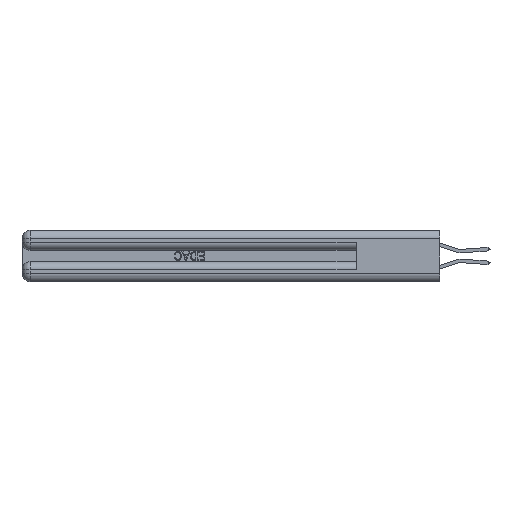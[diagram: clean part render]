
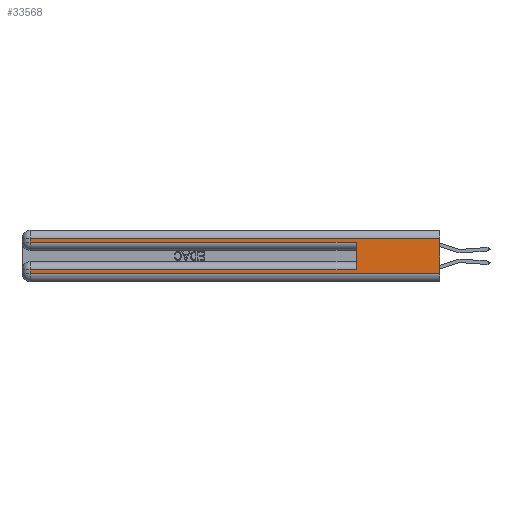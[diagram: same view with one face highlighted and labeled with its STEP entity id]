
A CAD part, left-side view. The second image highlights one B-rep face of the part: STEP entity #33568.
In plain terms, the highlighted planar face has unit normal (-1, 0, 0).
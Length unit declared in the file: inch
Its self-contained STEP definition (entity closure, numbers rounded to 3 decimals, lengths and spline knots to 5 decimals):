
#102 = CARTESIAN_POINT ( 'NONE',  ( 0., 0., 0.37 ) ) ;
#233 = EDGE_CURVE ( 'NONE', #40663, #16151, #23575, .T. ) ;
#331 = EDGE_LOOP ( 'NONE', ( #36158, #1715, #20571, #21414, #36851, #10045, #33916, #22500 ) ) ;
#1715 = ORIENTED_EDGE ( 'NONE', *, *, #34151, .T. ) ;
#2573 = PLANE ( 'NONE',  #15034 ) ;
#2609 = CARTESIAN_POINT ( 'NONE',  ( 0., 0.6, 0.285 ) ) ;
#2810 = VECTOR ( 'NONE', #10468, 39.37008 ) ;
#4701 = VERTEX_POINT ( 'NONE', #22390 ) ;
#4726 = CARTESIAN_POINT ( 'NONE',  ( 0., 0., 0.31 ) ) ;
#4946 = VECTOR ( 'NONE', #12171, 39.37008 ) ;
#5320 = LINE ( 'NONE', #102, #11819 ) ;
#5517 = FACE_OUTER_BOUND ( 'NONE', #331, .T. ) ;
#5545 = VECTOR ( 'NONE', #16810, 39.37008 ) ;
#6520 = CARTESIAN_POINT ( 'NONE',  ( 0., 2.94, 0.085 ) ) ;
#7369 = VERTEX_POINT ( 'NONE', #13444 ) ;
#7971 = VECTOR ( 'NONE', #37276, 39.37008 ) ;
#9285 = CARTESIAN_POINT ( 'NONE',  ( 0., 2.94, 0.31 ) ) ;
#9429 = CARTESIAN_POINT ( 'NONE',  ( 0., 2.94, 0.37 ) ) ;
#10045 = ORIENTED_EDGE ( 'NONE', *, *, #20470, .T. ) ;
#10185 = LINE ( 'NONE', #15118, #29690 ) ;
#10468 = DIRECTION ( 'NONE',  ( 0., -1., 0. ) ) ;
#11209 = VERTEX_POINT ( 'NONE', #2609 ) ;
#11819 = VECTOR ( 'NONE', #30062, 39.37008 ) ;
#12171 = DIRECTION ( 'NONE',  ( 0., 1., 0. ) ) ;
#13444 = CARTESIAN_POINT ( 'NONE',  ( 0., 0., 0.31 ) ) ;
#14262 = CARTESIAN_POINT ( 'NONE',  ( 0., 2.94, 0.285 ) ) ;
#14694 = VECTOR ( 'NONE', #25781, 39.37008 ) ;
#15031 = EDGE_CURVE ( 'NONE', #39409, #11209, #10185, .T. ) ;
#15034 = AXIS2_PLACEMENT_3D ( 'NONE', #15202, #18290, #40690 ) ;
#15118 = CARTESIAN_POINT ( 'NONE',  ( 0., 0.6, 0.145 ) ) ;
#15202 = CARTESIAN_POINT ( 'NONE',  ( 0., 0., 0.37 ) ) ;
#15483 = LINE ( 'NONE', #34781, #4946 ) ;
#16151 = VERTEX_POINT ( 'NONE', #14262 ) ;
#16810 = DIRECTION ( 'NONE',  ( 0., 0., -1. ) ) ;
#18290 = DIRECTION ( 'NONE',  ( 1., 0., 0. ) ) ;
#19705 = VERTEX_POINT ( 'NONE', #39984 ) ;
#20339 = EDGE_CURVE ( 'NONE', #31127, #4701, #27033, .T. ) ;
#20470 = EDGE_CURVE ( 'NONE', #39409, #31127, #15483, .T. ) ;
#20571 = ORIENTED_EDGE ( 'NONE', *, *, #233, .T. ) ;
#21414 = ORIENTED_EDGE ( 'NONE', *, *, #28844, .T. ) ;
#22286 = EDGE_CURVE ( 'NONE', #4701, #19705, #28364, .T. ) ;
#22390 = CARTESIAN_POINT ( 'NONE',  ( 0., 2.94, 0.06 ) ) ;
#22500 = ORIENTED_EDGE ( 'NONE', *, *, #22286, .T. ) ;
#22824 = CARTESIAN_POINT ( 'NONE',  ( 0., 0., 0.285 ) ) ;
#23225 = CARTESIAN_POINT ( 'NONE',  ( 0., 0., 0.06 ) ) ;
#23575 = LINE ( 'NONE', #9429, #5545 ) ;
#25781 = DIRECTION ( 'NONE',  ( 0., -1., 0. ) ) ;
#27033 = LINE ( 'NONE', #40493, #7971 ) ;
#28364 = LINE ( 'NONE', #23225, #2810 ) ;
#28844 = EDGE_CURVE ( 'NONE', #16151, #11209, #33801, .T. ) ;
#29632 = DIRECTION ( 'NONE',  ( 0., 1., 0. ) ) ;
#29690 = VECTOR ( 'NONE', #37531, 39.37008 ) ;
#30062 = DIRECTION ( 'NONE',  ( 0., 0., -1. ) ) ;
#31127 = VERTEX_POINT ( 'NONE', #6520 ) ;
#32525 = VECTOR ( 'NONE', #29632, 39.37008 ) ;
#33568 = ADVANCED_FACE ( 'NONE', ( #5517 ), #2573, .F. ) ;
#33801 = LINE ( 'NONE', #22824, #14694 ) ;
#33916 = ORIENTED_EDGE ( 'NONE', *, *, #20339, .T. ) ;
#34094 = LINE ( 'NONE', #4726, #32525 ) ;
#34151 = EDGE_CURVE ( 'NONE', #7369, #40663, #34094, .T. ) ;
#34781 = CARTESIAN_POINT ( 'NONE',  ( 0., 0., 0.085 ) ) ;
#36007 = EDGE_CURVE ( 'NONE', #7369, #19705, #5320, .T. ) ;
#36158 = ORIENTED_EDGE ( 'NONE', *, *, #36007, .F. ) ;
#36851 = ORIENTED_EDGE ( 'NONE', *, *, #15031, .F. ) ;
#37276 = DIRECTION ( 'NONE',  ( 0., 0., -1. ) ) ;
#37457 = CARTESIAN_POINT ( 'NONE',  ( 0., 0.6, 0.085 ) ) ;
#37531 = DIRECTION ( 'NONE',  ( 0., 0., 1. ) ) ;
#39409 = VERTEX_POINT ( 'NONE', #37457 ) ;
#39984 = CARTESIAN_POINT ( 'NONE',  ( 0., 0., 0.06 ) ) ;
#40493 = CARTESIAN_POINT ( 'NONE',  ( 0., 2.94, 0.37 ) ) ;
#40663 = VERTEX_POINT ( 'NONE', #9285 ) ;
#40690 = DIRECTION ( 'NONE',  ( 0., 0., -1. ) ) ;
